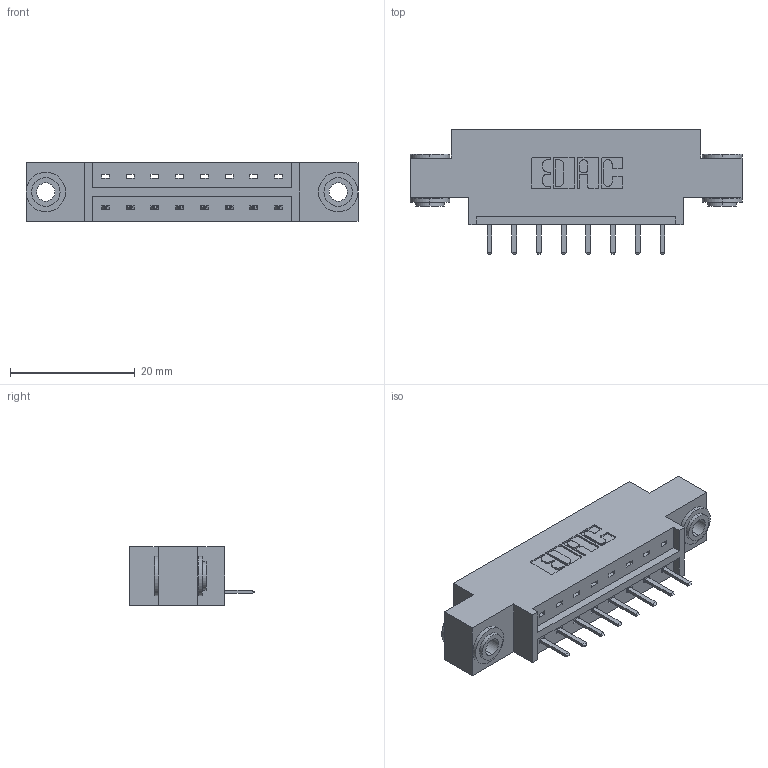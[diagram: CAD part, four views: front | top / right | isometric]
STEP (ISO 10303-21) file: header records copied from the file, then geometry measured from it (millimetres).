
FILE_DESCRIPTION (( 'STEP AP203' ), '1' );
FILE_NAME ('333-008-520-603.STEP', '2018-07-31T21:55:03', ( '' ), ( '' ), 'SwSTEP 2.0', 'SolidWorks 2016', '' );
FILE_SCHEMA (( 'CONFIG_CONTROL_DESIGN' ));
Length unit declared in the file: inch
Products named in the file (4): 345-292-001_345-293-120; 345-250-002_345-250-002-102; 333-008-520-603; 333 Part_Offset - .156 Dia - TH
Assembly tree (11 placements, depth 2):
  333-008-520-603
    333 Part_Offset - .156 Dia - TH
    345-292-001_345-293-120  x8
    345-250-002_345-250-002-102  x2
Bounding box: 53.24 x 20.02 x 9.4 mm (x, y, z)
Volume: 4833.5 mm3; surface area: 5352 mm2
Topology: 11 solids, 11 shells, 652 faces, 1871 edges, 1222 vertices
Faces by surface type: plane 436, cylinder 208, cone 8
Entity records: 10184 total; most frequent: CARTESIAN_POINT 1753, ORIENTED_EDGE 1678, DIRECTION 1569, EDGE_CURVE 839, LINE 683, VECTOR 683, VERTEX_POINT 554, AXIS2_PLACEMENT_3D 443
